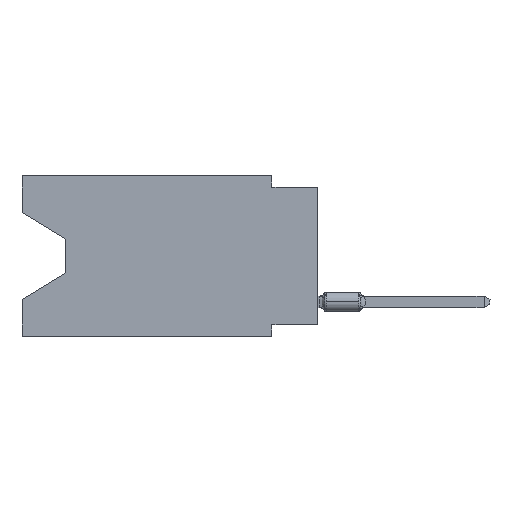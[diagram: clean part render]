
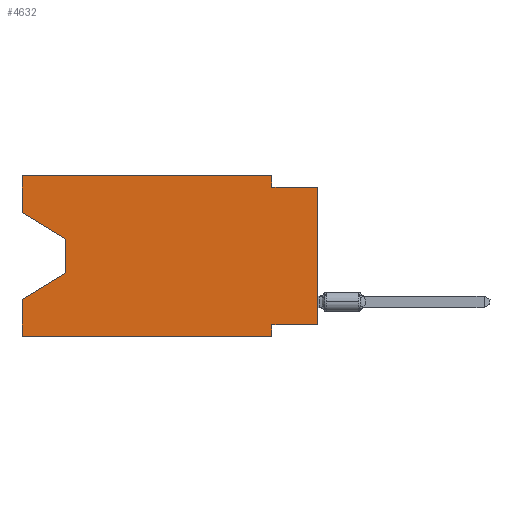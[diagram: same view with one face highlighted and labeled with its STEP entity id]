
A CAD part, left-side view. The second image highlights one B-rep face of the part: STEP entity #4632.
In plain terms, the highlighted planar face has unit normal (-1, 0, 0).
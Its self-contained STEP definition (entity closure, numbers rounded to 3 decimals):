
#125 = CARTESIAN_POINT ( 'NONE',  ( 0., 0., -8.255 ) ) ;
#822 = VECTOR ( 'NONE', #15968, 1000. ) ;
#952 = VERTEX_POINT ( 'NONE', #24152 ) ;
#1098 = CARTESIAN_POINT ( 'NONE',  ( 0., 13.97, -5.385 ) ) ;
#1472 = EDGE_CURVE ( 'NONE', #24887, #8425, #8457, .T. ) ;
#1861 = EDGE_LOOP ( 'NONE', ( #8576, #20381, #8514, #18195, #3948, #8882, #28492, #2269, #6046, #20608, #27540, #13710 ) ) ;
#2033 = FACE_OUTER_BOUND ( 'NONE', #1861, .T. ) ;
#2269 = ORIENTED_EDGE ( 'NONE', *, *, #7094, .T. ) ;
#3033 = LINE ( 'NONE', #12294, #26519 ) ;
#3948 = ORIENTED_EDGE ( 'NONE', *, *, #11315, .T. ) ;
#4594 = CARTESIAN_POINT ( 'NONE',  ( 0., 16.383, 0. ) ) ;
#4632 = ADVANCED_FACE ( 'NONE', ( #2033 ), #29507, .F. ) ;
#5077 = CARTESIAN_POINT ( 'NONE',  ( 0., 16.383, -6.852 ) ) ;
#5718 = CARTESIAN_POINT ( 'NONE',  ( 0., 2.54, -8.255 ) ) ;
#5834 = LINE ( 'NONE', #13268, #17075 ) ;
#6046 = ORIENTED_EDGE ( 'NONE', *, *, #20765, .F. ) ;
#6285 = DIRECTION ( 'NONE',  ( 0., 0., -1. ) ) ;
#6705 = CARTESIAN_POINT ( 'NONE',  ( 0., 16.383, 0. ) ) ;
#7094 = EDGE_CURVE ( 'NONE', #21575, #22634, #29927, .T. ) ;
#7476 = CARTESIAN_POINT ( 'NONE',  ( 0., 0., -0.635 ) ) ;
#8190 = EDGE_CURVE ( 'NONE', #952, #20390, #22336, .T. ) ;
#8396 = VECTOR ( 'NONE', #9751, 1000. ) ;
#8425 = VERTEX_POINT ( 'NONE', #13952 ) ;
#8457 = LINE ( 'NONE', #18048, #21320 ) ;
#8514 = ORIENTED_EDGE ( 'NONE', *, *, #25229, .T. ) ;
#8540 = VERTEX_POINT ( 'NONE', #9532 ) ;
#8576 = ORIENTED_EDGE ( 'NONE', *, *, #1472, .T. ) ;
#8578 = DIRECTION ( 'NONE',  ( 0., -1., 0. ) ) ;
#8666 = CARTESIAN_POINT ( 'NONE',  ( 0., 16.383, -2.038 ) ) ;
#8709 = LINE ( 'NONE', #15832, #25269 ) ;
#8882 = ORIENTED_EDGE ( 'NONE', *, *, #18279, .F. ) ;
#9532 = CARTESIAN_POINT ( 'NONE',  ( 0., 2.54, -8.89 ) ) ;
#9751 = DIRECTION ( 'NONE',  ( 0., -1., 0. ) ) ;
#9798 = VERTEX_POINT ( 'NONE', #29491 ) ;
#9829 = CARTESIAN_POINT ( 'NONE',  ( 0., 2.54, -0.635 ) ) ;
#9860 = VECTOR ( 'NONE', #15518, 1000. ) ;
#10172 = EDGE_CURVE ( 'NONE', #14648, #952, #29631, .T. ) ;
#10487 = DIRECTION ( 'NONE',  ( 0., 0.855, -0.519 ) ) ;
#10588 = DIRECTION ( 'NONE',  ( 0., -0.855, -0.519 ) ) ;
#11315 = EDGE_CURVE ( 'NONE', #9798, #8540, #29527, .T. ) ;
#12294 = CARTESIAN_POINT ( 'NONE',  ( 0., 2.54, -8.89 ) ) ;
#12766 = CARTESIAN_POINT ( 'NONE',  ( 0., 2.54, 0. ) ) ;
#13268 = CARTESIAN_POINT ( 'NONE',  ( 0., 13.97, -3.505 ) ) ;
#13410 = CARTESIAN_POINT ( 'NONE',  ( 0., 16.383, 0. ) ) ;
#13442 = VECTOR ( 'NONE', #26746, 1000. ) ;
#13710 = ORIENTED_EDGE ( 'NONE', *, *, #25161, .F. ) ;
#13952 = CARTESIAN_POINT ( 'NONE',  ( 0., 13.97, -3.505 ) ) ;
#14648 = VERTEX_POINT ( 'NONE', #27164 ) ;
#15518 = DIRECTION ( 'NONE',  ( 0., 1., 0. ) ) ;
#15832 = CARTESIAN_POINT ( 'NONE',  ( 0., 16.383, 0. ) ) ;
#15968 = DIRECTION ( 'NONE',  ( 0., -1., 0. ) ) ;
#16432 = DIRECTION ( 'NONE',  ( 0., 0., 1. ) ) ;
#16686 = VERTEX_POINT ( 'NONE', #5718 ) ;
#17075 = VECTOR ( 'NONE', #6285, 1000. ) ;
#17668 = LINE ( 'NONE', #22656, #9860 ) ;
#17690 = CARTESIAN_POINT ( 'NONE',  ( 0., 13.97, -5.385 ) ) ;
#17777 = VECTOR ( 'NONE', #25391, 1000. ) ;
#18048 = CARTESIAN_POINT ( 'NONE',  ( 0., 16.383, -2.038 ) ) ;
#18195 = ORIENTED_EDGE ( 'NONE', *, *, #22361, .F. ) ;
#18279 = EDGE_CURVE ( 'NONE', #16686, #8540, #3033, .T. ) ;
#18884 = LINE ( 'NONE', #7476, #8396 ) ;
#19327 = VECTOR ( 'NONE', #16432, 1000. ) ;
#19340 = EDGE_CURVE ( 'NONE', #8425, #27884, #5834, .T. ) ;
#20381 = ORIENTED_EDGE ( 'NONE', *, *, #19340, .T. ) ;
#20390 = VERTEX_POINT ( 'NONE', #9829 ) ;
#20412 = DIRECTION ( 'NONE',  ( 1., 0., 0. ) ) ;
#20471 = DIRECTION ( 'NONE',  ( 0., 0., -1. ) ) ;
#20608 = ORIENTED_EDGE ( 'NONE', *, *, #8190, .F. ) ;
#20765 = EDGE_CURVE ( 'NONE', #20390, #22634, #18884, .T. ) ;
#20942 = EDGE_CURVE ( 'NONE', #21575, #16686, #17668, .T. ) ;
#21320 = VECTOR ( 'NONE', #10588, 1000. ) ;
#21575 = VERTEX_POINT ( 'NONE', #125 ) ;
#22336 = LINE ( 'NONE', #12766, #13442 ) ;
#22361 = EDGE_CURVE ( 'NONE', #9798, #27733, #8709, .T. ) ;
#22634 = VERTEX_POINT ( 'NONE', #28570 ) ;
#22656 = CARTESIAN_POINT ( 'NONE',  ( 0., 0., -8.255 ) ) ;
#22986 = DIRECTION ( 'NONE',  ( 0., 0., 1. ) ) ;
#24152 = CARTESIAN_POINT ( 'NONE',  ( 0., 2.54, 0. ) ) ;
#24326 = LINE ( 'NONE', #1098, #27562 ) ;
#24887 = VERTEX_POINT ( 'NONE', #8666 ) ;
#25161 = EDGE_CURVE ( 'NONE', #24887, #14648, #25984, .T. ) ;
#25229 = EDGE_CURVE ( 'NONE', #27884, #27733, #24326, .T. ) ;
#25269 = VECTOR ( 'NONE', #22986, 1000. ) ;
#25391 = DIRECTION ( 'NONE',  ( 0., 0., 1. ) ) ;
#25984 = LINE ( 'NONE', #4594, #19327 ) ;
#26519 = VECTOR ( 'NONE', #20471, 1000. ) ;
#26746 = DIRECTION ( 'NONE',  ( 0., 0., -1. ) ) ;
#26944 = DIRECTION ( 'NONE',  ( 0., 0., -1. ) ) ;
#27164 = CARTESIAN_POINT ( 'NONE',  ( 0., 16.383, 0. ) ) ;
#27540 = ORIENTED_EDGE ( 'NONE', *, *, #10172, .F. ) ;
#27562 = VECTOR ( 'NONE', #10487, 1000. ) ;
#27680 = AXIS2_PLACEMENT_3D ( 'NONE', #13410, #20412, #26944 ) ;
#27733 = VERTEX_POINT ( 'NONE', #5077 ) ;
#27884 = VERTEX_POINT ( 'NONE', #17690 ) ;
#28100 = CARTESIAN_POINT ( 'NONE',  ( 0., 0., 0. ) ) ;
#28350 = VECTOR ( 'NONE', #8578, 1000. ) ;
#28492 = ORIENTED_EDGE ( 'NONE', *, *, #20942, .F. ) ;
#28570 = CARTESIAN_POINT ( 'NONE',  ( 0., 0., -0.635 ) ) ;
#29374 = CARTESIAN_POINT ( 'NONE',  ( 0., 16.383, -8.89 ) ) ;
#29491 = CARTESIAN_POINT ( 'NONE',  ( 0., 16.383, -8.89 ) ) ;
#29507 = PLANE ( 'NONE',  #27680 ) ;
#29527 = LINE ( 'NONE', #29374, #28350 ) ;
#29631 = LINE ( 'NONE', #6705, #822 ) ;
#29927 = LINE ( 'NONE', #28100, #17777 ) ;
